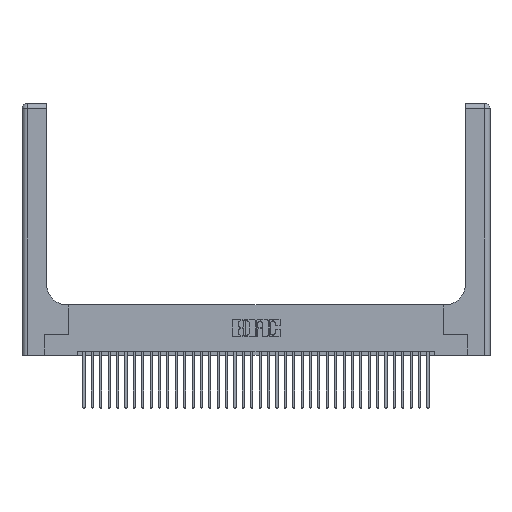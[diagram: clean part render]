
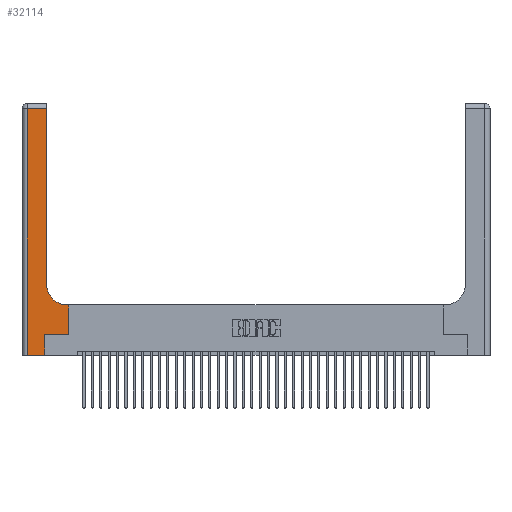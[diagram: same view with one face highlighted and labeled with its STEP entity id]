
A CAD part, top view. The second image highlights one B-rep face of the part: STEP entity #32114.
In plain terms, the highlighted planar face has unit normal (0, 0, 1).
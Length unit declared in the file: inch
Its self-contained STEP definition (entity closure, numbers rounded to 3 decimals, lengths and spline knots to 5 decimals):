
#1689 = VERTEX_POINT ( 'NONE', #14720 ) ;
#1701 = CARTESIAN_POINT ( 'NONE',  ( 0.269, 0., 0.37 ) ) ;
#2623 = ORIENTED_EDGE ( 'NONE', *, *, #21377, .T. ) ;
#2649 = LINE ( 'NONE', #33942, #25322 ) ;
#3559 = CARTESIAN_POINT ( 'NONE',  ( 0.269, 0.25, 0.37 ) ) ;
#4913 = CARTESIAN_POINT ( 'NONE',  ( 0.5585, 0.6, 0.37 ) ) ;
#4997 = EDGE_CURVE ( 'NONE', #31430, #7773, #26686, .T. ) ;
#5915 = VERTEX_POINT ( 'NONE', #9375 ) ;
#6514 = CARTESIAN_POINT ( 'NONE',  ( 0.5585, 0.25, 0.37 ) ) ;
#7207 = CARTESIAN_POINT ( 'NONE',  ( 0.5415, 0.85, 0.37 ) ) ;
#7511 = EDGE_CURVE ( 'NONE', #15169, #17688, #21887, .T. ) ;
#7773 = VERTEX_POINT ( 'NONE', #32817 ) ;
#8966 = VECTOR ( 'NONE', #29699, 39.37008 ) ;
#8997 = ORIENTED_EDGE ( 'NONE', *, *, #31173, .T. ) ;
#9375 = CARTESIAN_POINT ( 'NONE',  ( 0.5415, 0.6, 0.37 ) ) ;
#9440 = CARTESIAN_POINT ( 'NONE',  ( 0., 3., 0.37 ) ) ;
#10134 = CARTESIAN_POINT ( 'NONE',  ( 0.2915, 3., 0.37 ) ) ;
#10207 = DIRECTION ( 'NONE',  ( 1., 0., 0. ) ) ;
#10942 = DIRECTION ( 'NONE',  ( 0., -1., 0. ) ) ;
#11376 = CARTESIAN_POINT ( 'NONE',  ( 0.5585, 0.25, 0.37 ) ) ;
#11738 = LINE ( 'NONE', #17858, #8966 ) ;
#11930 = VECTOR ( 'NONE', #27209, 39.37008 ) ;
#12413 = DIRECTION ( 'NONE',  ( -1., 0., 0. ) ) ;
#12774 = AXIS2_PLACEMENT_3D ( 'NONE', #9440, #30076, #12413 ) ;
#14720 = CARTESIAN_POINT ( 'NONE',  ( 0.269, 0.25, 0.37 ) ) ;
#14765 = EDGE_CURVE ( 'NONE', #37364, #1689, #26765, .T. ) ;
#14802 = ORIENTED_EDGE ( 'NONE', *, *, #14765, .T. ) ;
#15165 = EDGE_LOOP ( 'NONE', ( #29935, #8997, #37994, #31841, #14802, #2623, #35710, #24879, #33333 ) ) ;
#15169 = VERTEX_POINT ( 'NONE', #19309 ) ;
#16797 = VERTEX_POINT ( 'NONE', #6514 ) ;
#17321 = DIRECTION ( 'NONE',  ( 0., 1., 0. ) ) ;
#17364 = EDGE_CURVE ( 'NONE', #17688, #37364, #11738, .T. ) ;
#17688 = VERTEX_POINT ( 'NONE', #34008 ) ;
#17858 = CARTESIAN_POINT ( 'NONE',  ( 0., 0., 0.37 ) ) ;
#17918 = EDGE_CURVE ( 'NONE', #30129, #5915, #37480, .T. ) ;
#18022 = CARTESIAN_POINT ( 'NONE',  ( 0.2915, 0.85, 0.37 ) ) ;
#18947 = VECTOR ( 'NONE', #22806, 39.37008 ) ;
#19309 = CARTESIAN_POINT ( 'NONE',  ( 0.06, 2.94, 0.37 ) ) ;
#21097 = EDGE_CURVE ( 'NONE', #16797, #30129, #37748, .T. ) ;
#21377 = EDGE_CURVE ( 'NONE', #1689, #16797, #27627, .T. ) ;
#21887 = LINE ( 'NONE', #37341, #35655 ) ;
#22806 = DIRECTION ( 'NONE',  ( 0., 1., 0. ) ) ;
#24879 = ORIENTED_EDGE ( 'NONE', *, *, #17918, .T. ) ;
#25322 = VECTOR ( 'NONE', #28068, 39.37008 ) ;
#26686 = LINE ( 'NONE', #10134, #34472 ) ;
#26765 = LINE ( 'NONE', #31544, #18947 ) ;
#27102 = PLANE ( 'NONE',  #12774 ) ;
#27209 = DIRECTION ( 'NONE',  ( 1., 0., 0. ) ) ;
#27627 = LINE ( 'NONE', #3559, #11930 ) ;
#27872 = DIRECTION ( 'NONE',  ( 0., 0., -1. ) ) ;
#28068 = DIRECTION ( 'NONE',  ( -1., 0., 0. ) ) ;
#28317 = CARTESIAN_POINT ( 'NONE',  ( 0.2915, 0.6, 0.37 ) ) ;
#29680 = VECTOR ( 'NONE', #31247, 39.37008 ) ;
#29699 = DIRECTION ( 'NONE',  ( 1., 0., 0. ) ) ;
#29935 = ORIENTED_EDGE ( 'NONE', *, *, #4997, .T. ) ;
#29952 = VECTOR ( 'NONE', #17321, 39.37008 ) ;
#30076 = DIRECTION ( 'NONE',  ( 0., 0., -1. ) ) ;
#30129 = VERTEX_POINT ( 'NONE', #4913 ) ;
#30757 = DIRECTION ( 'NONE',  ( 0., 1., 0. ) ) ;
#31173 = EDGE_CURVE ( 'NONE', #7773, #15169, #2649, .T. ) ;
#31247 = DIRECTION ( 'NONE',  ( -1., 0., 0. ) ) ;
#31430 = VERTEX_POINT ( 'NONE', #18022 ) ;
#31544 = CARTESIAN_POINT ( 'NONE',  ( 0.269, 0., 0.37 ) ) ;
#31547 = CIRCLE ( 'NONE', #32065, 0.25 ) ;
#31841 = ORIENTED_EDGE ( 'NONE', *, *, #17364, .T. ) ;
#32065 = AXIS2_PLACEMENT_3D ( 'NONE', #7207, #27872, #10207 ) ;
#32114 = ADVANCED_FACE ( 'NONE', ( #33550 ), #27102, .F. ) ;
#32817 = CARTESIAN_POINT ( 'NONE',  ( 0.2915, 2.94, 0.37 ) ) ;
#33333 = ORIENTED_EDGE ( 'NONE', *, *, #34485, .T. ) ;
#33550 = FACE_OUTER_BOUND ( 'NONE', #15165, .T. ) ;
#33942 = CARTESIAN_POINT ( 'NONE',  ( 0., 2.94, 0.37 ) ) ;
#34008 = CARTESIAN_POINT ( 'NONE',  ( 0.06, 0., 0.37 ) ) ;
#34472 = VECTOR ( 'NONE', #30757, 39.37008 ) ;
#34485 = EDGE_CURVE ( 'NONE', #5915, #31430, #31547, .T. ) ;
#35655 = VECTOR ( 'NONE', #10942, 39.37008 ) ;
#35710 = ORIENTED_EDGE ( 'NONE', *, *, #21097, .T. ) ;
#37341 = CARTESIAN_POINT ( 'NONE',  ( 0.06, 3., 0.37 ) ) ;
#37364 = VERTEX_POINT ( 'NONE', #1701 ) ;
#37480 = LINE ( 'NONE', #28317, #29680 ) ;
#37748 = LINE ( 'NONE', #11376, #29952 ) ;
#37994 = ORIENTED_EDGE ( 'NONE', *, *, #7511, .T. ) ;
